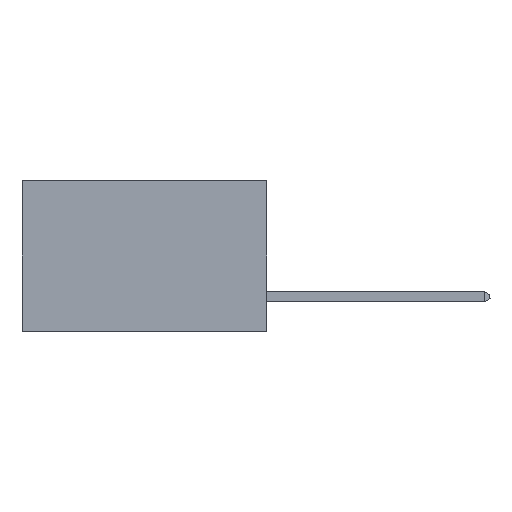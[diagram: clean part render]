
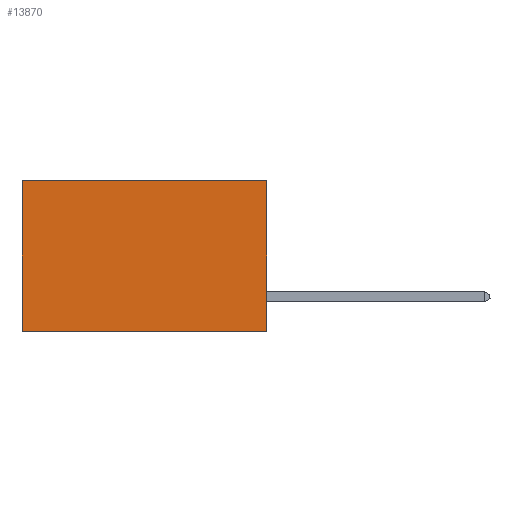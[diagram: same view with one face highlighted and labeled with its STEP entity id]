
A CAD part, left-side view. The second image highlights one B-rep face of the part: STEP entity #13870.
In plain terms, the highlighted planar face has unit normal (-1, 0, 0).
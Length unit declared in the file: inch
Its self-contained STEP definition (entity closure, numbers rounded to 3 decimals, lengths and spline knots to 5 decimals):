
#1617 = DIRECTION ( 'NONE',  ( 0., 1., 0. ) ) ;
#2909 = LINE ( 'NONE', #6884, #11320 ) ;
#3138 = LINE ( 'NONE', #16999, #13453 ) ;
#3929 = ORIENTED_EDGE ( 'NONE', *, *, #4358, .T. ) ;
#3980 = CARTESIAN_POINT ( 'NONE',  ( 0.2875, 0.6, -0.37 ) ) ;
#4358 = EDGE_CURVE ( 'NONE', #5475, #21408, #2909, .T. ) ;
#4589 = EDGE_CURVE ( 'NONE', #24684, #15376, #20986, .T. ) ;
#4811 = DIRECTION ( 'NONE',  ( 0., 0., -1. ) ) ;
#5152 = CARTESIAN_POINT ( 'NONE',  ( 0.2875, 0., 0. ) ) ;
#5475 = VERTEX_POINT ( 'NONE', #10908 ) ;
#6884 = CARTESIAN_POINT ( 'NONE',  ( 0.2875, 0., 0. ) ) ;
#6991 = ORIENTED_EDGE ( 'NONE', *, *, #4589, .F. ) ;
#9904 = EDGE_CURVE ( 'NONE', #21408, #15376, #24888, .T. ) ;
#10403 = VECTOR ( 'NONE', #1617, 39.37008 ) ;
#10690 = CARTESIAN_POINT ( 'NONE',  ( 0.2875, 0.6, 0. ) ) ;
#10908 = CARTESIAN_POINT ( 'NONE',  ( 0.2875, 0., 0. ) ) ;
#11320 = VECTOR ( 'NONE', #20781, 39.37008 ) ;
#13453 = VECTOR ( 'NONE', #15072, 39.37008 ) ;
#13477 = CARTESIAN_POINT ( 'NONE',  ( 0.2875, 0., -0.37 ) ) ;
#13851 = EDGE_LOOP ( 'NONE', ( #23844, #6991, #22656, #3929 ) ) ;
#13870 = ADVANCED_FACE ( 'NONE', ( #20199 ), #23009, .F. ) ;
#14534 = DIRECTION ( 'NONE',  ( 0., 0., -1. ) ) ;
#15072 = DIRECTION ( 'NONE',  ( 0., 0., -1. ) ) ;
#15376 = VERTEX_POINT ( 'NONE', #3980 ) ;
#16760 = DIRECTION ( 'NONE',  ( 1., 0., 0. ) ) ;
#16929 = AXIS2_PLACEMENT_3D ( 'NONE', #5152, #16760, #4811 ) ;
#16999 = CARTESIAN_POINT ( 'NONE',  ( 0.2875, 0., 0. ) ) ;
#17404 = EDGE_CURVE ( 'NONE', #5475, #24684, #3138, .T. ) ;
#20199 = FACE_OUTER_BOUND ( 'NONE', #13851, .T. ) ;
#20781 = DIRECTION ( 'NONE',  ( 0., 1., 0. ) ) ;
#20986 = LINE ( 'NONE', #13477, #10403 ) ;
#21408 = VERTEX_POINT ( 'NONE', #22269 ) ;
#22269 = CARTESIAN_POINT ( 'NONE',  ( 0.2875, 0.6, 0. ) ) ;
#22386 = VECTOR ( 'NONE', #14534, 39.37008 ) ;
#22656 = ORIENTED_EDGE ( 'NONE', *, *, #17404, .F. ) ;
#23009 = PLANE ( 'NONE',  #16929 ) ;
#23684 = CARTESIAN_POINT ( 'NONE',  ( 0.2875, 0., -0.37 ) ) ;
#23844 = ORIENTED_EDGE ( 'NONE', *, *, #9904, .T. ) ;
#24684 = VERTEX_POINT ( 'NONE', #23684 ) ;
#24888 = LINE ( 'NONE', #10690, #22386 ) ;
